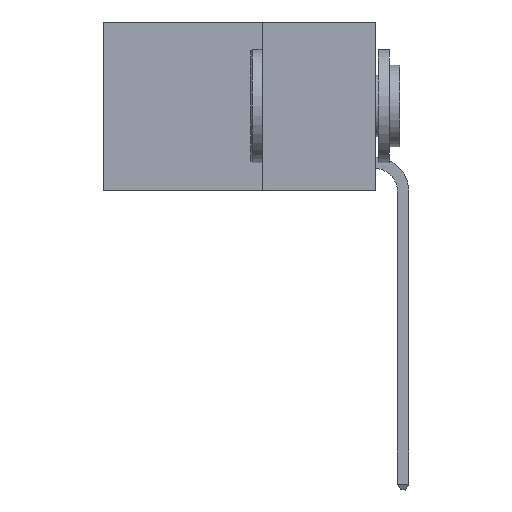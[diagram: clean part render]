
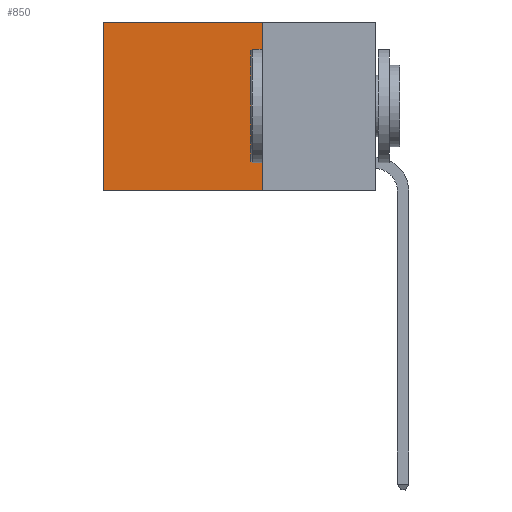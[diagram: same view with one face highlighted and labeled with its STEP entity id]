
A CAD part, left-side view. The second image highlights one B-rep face of the part: STEP entity #850.
In plain terms, the highlighted planar face has unit normal (-1, 0, 0).
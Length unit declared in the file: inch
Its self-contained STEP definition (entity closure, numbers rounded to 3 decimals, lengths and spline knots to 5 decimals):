
#87 = VERTEX_POINT ( 'NONE', #8799 ) ;
#218 = VECTOR ( 'NONE', #7155, 39.37008 ) ;
#270 = VECTOR ( 'NONE', #3229, 39.37008 ) ;
#295 = CARTESIAN_POINT ( 'NONE',  ( 0.2625, 0.6, -0.37 ) ) ;
#418 = EDGE_CURVE ( 'NONE', #87, #5552, #6879, .T. ) ;
#581 = VECTOR ( 'NONE', #4305, 39.37008 ) ;
#850 = ADVANCED_FACE ( 'NONE', ( #3018 ), #10295, .F. ) ;
#1758 = ORIENTED_EDGE ( 'NONE', *, *, #7062, .T. ) ;
#2791 = LINE ( 'NONE', #7523, #581 ) ;
#2929 = AXIS2_PLACEMENT_3D ( 'NONE', #3400, #5068, #4697 ) ;
#3018 = FACE_OUTER_BOUND ( 'NONE', #8623, .T. ) ;
#3115 = CARTESIAN_POINT ( 'NONE',  ( 0.2625, 0.6, 0. ) ) ;
#3229 = DIRECTION ( 'NONE',  ( 0., 1., 0. ) ) ;
#3381 = VERTEX_POINT ( 'NONE', #295 ) ;
#3400 = CARTESIAN_POINT ( 'NONE',  ( 0.2625, 0.25, 0. ) ) ;
#4305 = DIRECTION ( 'NONE',  ( 0., 0., -1. ) ) ;
#4697 = DIRECTION ( 'NONE',  ( 0., 0., -1. ) ) ;
#5068 = DIRECTION ( 'NONE',  ( 1., 0., 0. ) ) ;
#5471 = ORIENTED_EDGE ( 'NONE', *, *, #418, .T. ) ;
#5534 = CARTESIAN_POINT ( 'NONE',  ( 0.2625, 0.25, -0.37 ) ) ;
#5552 = VERTEX_POINT ( 'NONE', #3115 ) ;
#5600 = ORIENTED_EDGE ( 'NONE', *, *, #9719, .F. ) ;
#6278 = VERTEX_POINT ( 'NONE', #9967 ) ;
#6312 = ORIENTED_EDGE ( 'NONE', *, *, #10211, .F. ) ;
#6461 = LINE ( 'NONE', #8767, #218 ) ;
#6866 = VECTOR ( 'NONE', #9729, 39.37008 ) ;
#6879 = LINE ( 'NONE', #10093, #6866 ) ;
#7007 = LINE ( 'NONE', #5534, #270 ) ;
#7062 = EDGE_CURVE ( 'NONE', #5552, #3381, #6461, .T. ) ;
#7155 = DIRECTION ( 'NONE',  ( 0., 0., -1. ) ) ;
#7523 = CARTESIAN_POINT ( 'NONE',  ( 0.2625, 0.25, 0. ) ) ;
#8623 = EDGE_LOOP ( 'NONE', ( #1758, #6312, #5600, #5471 ) ) ;
#8767 = CARTESIAN_POINT ( 'NONE',  ( 0.2625, 0.6, 0. ) ) ;
#8799 = CARTESIAN_POINT ( 'NONE',  ( 0.2625, 0.25, 0. ) ) ;
#9719 = EDGE_CURVE ( 'NONE', #87, #6278, #2791, .T. ) ;
#9729 = DIRECTION ( 'NONE',  ( 0., 1., 0. ) ) ;
#9967 = CARTESIAN_POINT ( 'NONE',  ( 0.2625, 0.25, -0.37 ) ) ;
#10093 = CARTESIAN_POINT ( 'NONE',  ( 0.2625, 0.25, 0. ) ) ;
#10211 = EDGE_CURVE ( 'NONE', #6278, #3381, #7007, .T. ) ;
#10295 = PLANE ( 'NONE',  #2929 ) ;
